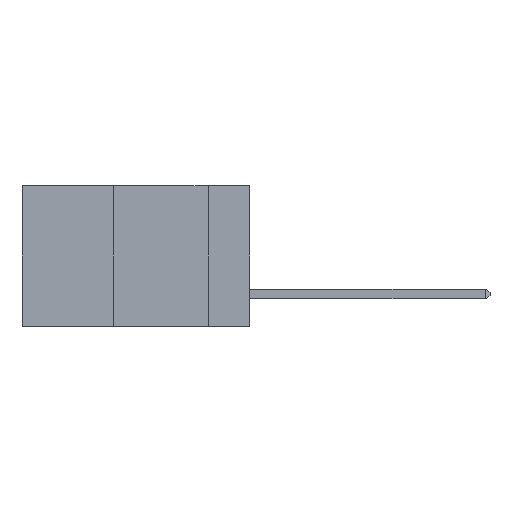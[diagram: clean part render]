
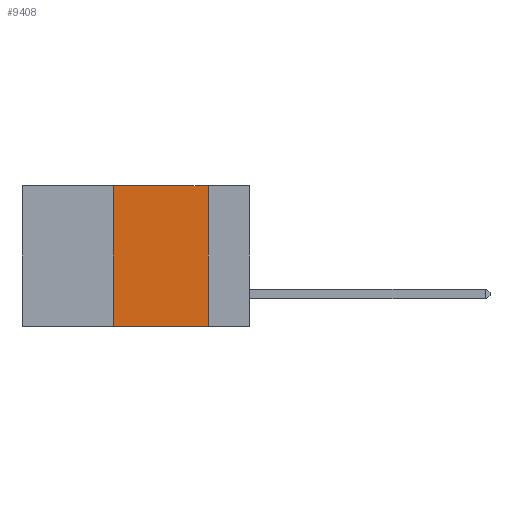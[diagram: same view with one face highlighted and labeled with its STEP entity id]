
A CAD part, left-side view. The second image highlights one B-rep face of the part: STEP entity #9408.
In plain terms, the highlighted planar face has unit normal (-1, 0, 0).
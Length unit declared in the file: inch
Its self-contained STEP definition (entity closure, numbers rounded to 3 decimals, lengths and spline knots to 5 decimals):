
#525 = EDGE_CURVE ( 'NONE', #6696, #14540, #15973, .T. ) ;
#2939 = CARTESIAN_POINT ( 'NONE',  ( 0., 0.36, 0. ) ) ;
#2954 = DIRECTION ( 'NONE',  ( 0., 0., 1. ) ) ;
#3210 = EDGE_LOOP ( 'NONE', ( #15922, #15985, #16299, #16485 ) ) ;
#4556 = VECTOR ( 'NONE', #5983, 39.37008 ) ;
#5168 = CARTESIAN_POINT ( 'NONE',  ( 0., 0.6, -0.37 ) ) ;
#5482 = EDGE_CURVE ( 'NONE', #14540, #9487, #8396, .T. ) ;
#5754 = EDGE_CURVE ( 'NONE', #6696, #6996, #14732, .T. ) ;
#5983 = DIRECTION ( 'NONE',  ( 0., -1., 0. ) ) ;
#6696 = VERTEX_POINT ( 'NONE', #8640 ) ;
#6996 = VERTEX_POINT ( 'NONE', #10751 ) ;
#7687 = AXIS2_PLACEMENT_3D ( 'NONE', #7853, #17605, #9280 ) ;
#7791 = PLANE ( 'NONE',  #7687 ) ;
#7853 = CARTESIAN_POINT ( 'NONE',  ( 0., 0.6, 0. ) ) ;
#8396 = LINE ( 'NONE', #8815, #4556 ) ;
#8640 = CARTESIAN_POINT ( 'NONE',  ( 0., 0.36, -0.37 ) ) ;
#8815 = CARTESIAN_POINT ( 'NONE',  ( 0., 0.6, 0. ) ) ;
#8927 = FACE_OUTER_BOUND ( 'NONE', #3210, .T. ) ;
#9014 = VECTOR ( 'NONE', #2954, 39.37008 ) ;
#9246 = CARTESIAN_POINT ( 'NONE',  ( 0., 0.11, 0. ) ) ;
#9280 = DIRECTION ( 'NONE',  ( 0., 0., -1. ) ) ;
#9408 = ADVANCED_FACE ( 'NONE', ( #8927 ), #7791, .F. ) ;
#9421 = LINE ( 'NONE', #9246, #12748 ) ;
#9426 = DIRECTION ( 'NONE',  ( 0., -1., 0. ) ) ;
#9487 = VERTEX_POINT ( 'NONE', #15008 ) ;
#10751 = CARTESIAN_POINT ( 'NONE',  ( 0., 0.11, -0.37 ) ) ;
#12748 = VECTOR ( 'NONE', #13426, 39.37008 ) ;
#13426 = DIRECTION ( 'NONE',  ( 0., 0., -1. ) ) ;
#14540 = VERTEX_POINT ( 'NONE', #15878 ) ;
#14732 = LINE ( 'NONE', #5168, #18385 ) ;
#15008 = CARTESIAN_POINT ( 'NONE',  ( 0., 0.11, 0. ) ) ;
#15878 = CARTESIAN_POINT ( 'NONE',  ( 0., 0.36, 0. ) ) ;
#15922 = ORIENTED_EDGE ( 'NONE', *, *, #16478, .F. ) ;
#15973 = LINE ( 'NONE', #2939, #9014 ) ;
#15985 = ORIENTED_EDGE ( 'NONE', *, *, #5482, .F. ) ;
#16299 = ORIENTED_EDGE ( 'NONE', *, *, #525, .F. ) ;
#16478 = EDGE_CURVE ( 'NONE', #9487, #6996, #9421, .T. ) ;
#16485 = ORIENTED_EDGE ( 'NONE', *, *, #5754, .T. ) ;
#17605 = DIRECTION ( 'NONE',  ( 1., 0., 0. ) ) ;
#18385 = VECTOR ( 'NONE', #9426, 39.37008 ) ;
